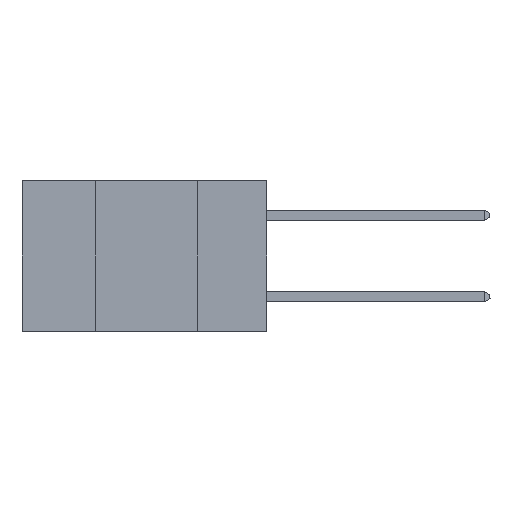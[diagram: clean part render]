
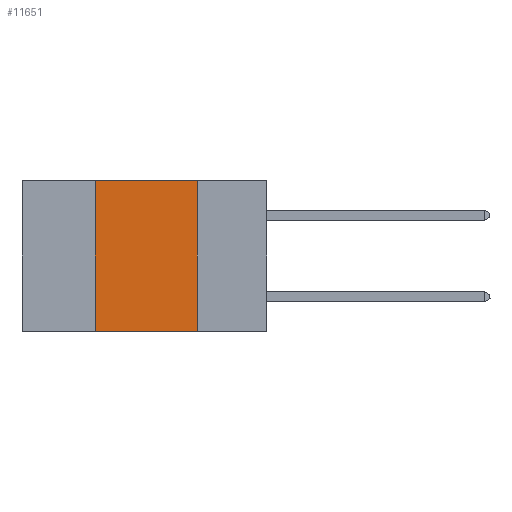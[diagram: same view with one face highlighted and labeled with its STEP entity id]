
A CAD part, left-side view. The second image highlights one B-rep face of the part: STEP entity #11651.
In plain terms, the highlighted planar face has unit normal (-1, 0, 0).
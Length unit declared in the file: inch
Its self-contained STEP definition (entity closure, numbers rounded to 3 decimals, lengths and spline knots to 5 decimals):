
#576 = ORIENTED_EDGE ( 'NONE', *, *, #5472, .T. ) ;
#814 = VECTOR ( 'NONE', #19783, 39.37008 ) ;
#2861 = FACE_OUTER_BOUND ( 'NONE', #41517, .T. ) ;
#3404 = VERTEX_POINT ( 'NONE', #19384 ) ;
#5472 = EDGE_CURVE ( 'NONE', #7418, #41419, #30152, .T. ) ;
#5635 = DIRECTION ( 'NONE',  ( 0., 0., -1. ) ) ;
#5659 = AXIS2_PLACEMENT_3D ( 'NONE', #16330, #6134, #30479 ) ;
#6134 = DIRECTION ( 'NONE',  ( 1., 0., 0. ) ) ;
#7203 = EDGE_CURVE ( 'NONE', #3404, #30573, #33165, .T. ) ;
#7418 = VERTEX_POINT ( 'NONE', #19958 ) ;
#8964 = LINE ( 'NONE', #43505, #35536 ) ;
#11307 = CARTESIAN_POINT ( 'NONE',  ( 0., 0.17, 0. ) ) ;
#11651 = ADVANCED_FACE ( 'NONE', ( #2861 ), #40616, .F. ) ;
#11846 = CARTESIAN_POINT ( 'NONE',  ( 0., 0.6, 0. ) ) ;
#13797 = VECTOR ( 'NONE', #33824, 39.37008 ) ;
#14727 = VECTOR ( 'NONE', #39518, 39.37008 ) ;
#15821 = ORIENTED_EDGE ( 'NONE', *, *, #7203, .F. ) ;
#16330 = CARTESIAN_POINT ( 'NONE',  ( 0., 0.6, 0. ) ) ;
#16579 = CARTESIAN_POINT ( 'NONE',  ( 0., 0.6, -0.37 ) ) ;
#19384 = CARTESIAN_POINT ( 'NONE',  ( 0., 0.42, 0. ) ) ;
#19783 = DIRECTION ( 'NONE',  ( 0., 0., 1. ) ) ;
#19958 = CARTESIAN_POINT ( 'NONE',  ( 0., 0.42, -0.37 ) ) ;
#27289 = ORIENTED_EDGE ( 'NONE', *, *, #41960, .F. ) ;
#27545 = LINE ( 'NONE', #40380, #814 ) ;
#29615 = EDGE_CURVE ( 'NONE', #30573, #41419, #8964, .T. ) ;
#30152 = LINE ( 'NONE', #16579, #13797 ) ;
#30479 = DIRECTION ( 'NONE',  ( 0., 0., -1. ) ) ;
#30573 = VERTEX_POINT ( 'NONE', #11307 ) ;
#33165 = LINE ( 'NONE', #11846, #14727 ) ;
#33170 = ORIENTED_EDGE ( 'NONE', *, *, #29615, .F. ) ;
#33824 = DIRECTION ( 'NONE',  ( 0., -1., 0. ) ) ;
#35536 = VECTOR ( 'NONE', #5635, 39.37008 ) ;
#39518 = DIRECTION ( 'NONE',  ( 0., -1., 0. ) ) ;
#40380 = CARTESIAN_POINT ( 'NONE',  ( 0., 0.42, 0. ) ) ;
#40616 = PLANE ( 'NONE',  #5659 ) ;
#41032 = CARTESIAN_POINT ( 'NONE',  ( 0., 0.17, -0.37 ) ) ;
#41419 = VERTEX_POINT ( 'NONE', #41032 ) ;
#41517 = EDGE_LOOP ( 'NONE', ( #33170, #15821, #27289, #576 ) ) ;
#41960 = EDGE_CURVE ( 'NONE', #7418, #3404, #27545, .T. ) ;
#43505 = CARTESIAN_POINT ( 'NONE',  ( 0., 0.17, 0. ) ) ;
